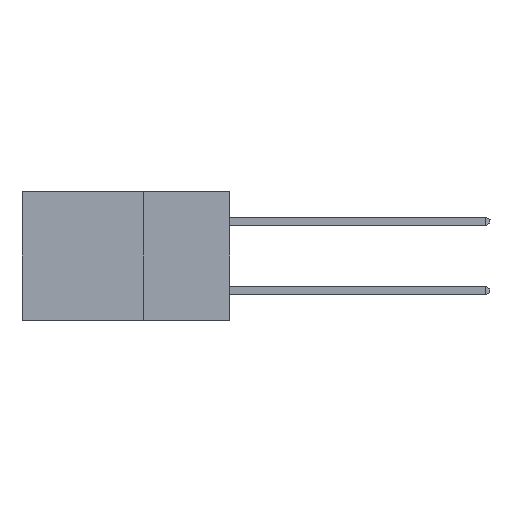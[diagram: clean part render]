
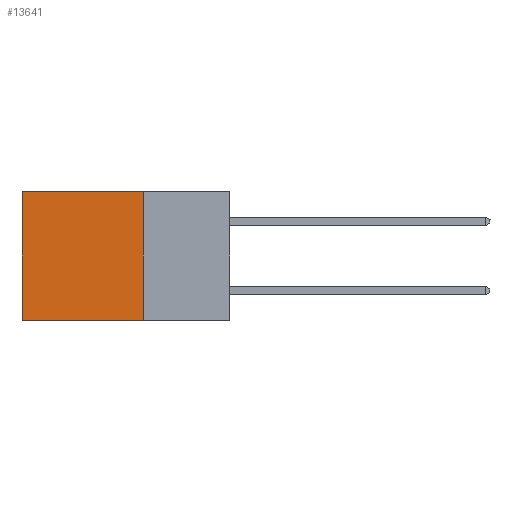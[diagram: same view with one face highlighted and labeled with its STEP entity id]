
A CAD part, left-side view. The second image highlights one B-rep face of the part: STEP entity #13641.
In plain terms, the highlighted planar face has unit normal (-1, 0, 0).
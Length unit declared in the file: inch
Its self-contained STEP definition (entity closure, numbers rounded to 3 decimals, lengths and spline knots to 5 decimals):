
#674 = PLANE ( 'NONE',  #20342 ) ;
#954 = EDGE_CURVE ( 'NONE', #21535, #20619, #10838, .T. ) ;
#2052 = DIRECTION ( 'NONE',  ( 1., 0., 0. ) ) ;
#2388 = VECTOR ( 'NONE', #3836, 39.37008 ) ;
#3746 = FACE_OUTER_BOUND ( 'NONE', #12263, .T. ) ;
#3836 = DIRECTION ( 'NONE',  ( 0., 1., 0. ) ) ;
#4314 = LINE ( 'NONE', #10764, #2388 ) ;
#4570 = LINE ( 'NONE', #13831, #22884 ) ;
#4859 = CARTESIAN_POINT ( 'NONE',  ( 0.298, 0.25, -0.37 ) ) ;
#6203 = VECTOR ( 'NONE', #19412, 39.37008 ) ;
#6838 = DIRECTION ( 'NONE',  ( 0., 0., -1. ) ) ;
#7493 = ORIENTED_EDGE ( 'NONE', *, *, #954, .F. ) ;
#8628 = EDGE_CURVE ( 'NONE', #21535, #22159, #4314, .T. ) ;
#10764 = CARTESIAN_POINT ( 'NONE',  ( 0.298, 0.25, 0. ) ) ;
#10838 = LINE ( 'NONE', #17646, #6203 ) ;
#11174 = CARTESIAN_POINT ( 'NONE',  ( 0.298, 0.25, 0. ) ) ;
#11441 = ORIENTED_EDGE ( 'NONE', *, *, #12273, .F. ) ;
#12263 = EDGE_LOOP ( 'NONE', ( #22697, #11441, #7493, #19385 ) ) ;
#12273 = EDGE_CURVE ( 'NONE', #20619, #20259, #21263, .T. ) ;
#13641 = ADVANCED_FACE ( 'NONE', ( #3746 ), #674, .F. ) ;
#13699 = CARTESIAN_POINT ( 'NONE',  ( 0.298, 0.6, -0.37 ) ) ;
#13738 = CARTESIAN_POINT ( 'NONE',  ( 0.298, 0.25, 0. ) ) ;
#13831 = CARTESIAN_POINT ( 'NONE',  ( 0.298, 0.6, 0. ) ) ;
#14459 = DIRECTION ( 'NONE',  ( 0., 0., -1. ) ) ;
#15395 = VECTOR ( 'NONE', #22372, 39.37008 ) ;
#16574 = CARTESIAN_POINT ( 'NONE',  ( 0.298, 0.6, 0. ) ) ;
#17646 = CARTESIAN_POINT ( 'NONE',  ( 0.298, 0.25, 0. ) ) ;
#19385 = ORIENTED_EDGE ( 'NONE', *, *, #8628, .T. ) ;
#19412 = DIRECTION ( 'NONE',  ( 0., 0., -1. ) ) ;
#20259 = VERTEX_POINT ( 'NONE', #13699 ) ;
#20342 = AXIS2_PLACEMENT_3D ( 'NONE', #11174, #2052, #14459 ) ;
#20619 = VERTEX_POINT ( 'NONE', #21686 ) ;
#21263 = LINE ( 'NONE', #4859, #15395 ) ;
#21535 = VERTEX_POINT ( 'NONE', #13738 ) ;
#21559 = EDGE_CURVE ( 'NONE', #22159, #20259, #4570, .T. ) ;
#21686 = CARTESIAN_POINT ( 'NONE',  ( 0.298, 0.25, -0.37 ) ) ;
#22159 = VERTEX_POINT ( 'NONE', #16574 ) ;
#22372 = DIRECTION ( 'NONE',  ( 0., 1., 0. ) ) ;
#22697 = ORIENTED_EDGE ( 'NONE', *, *, #21559, .T. ) ;
#22884 = VECTOR ( 'NONE', #6838, 39.37008 ) ;
